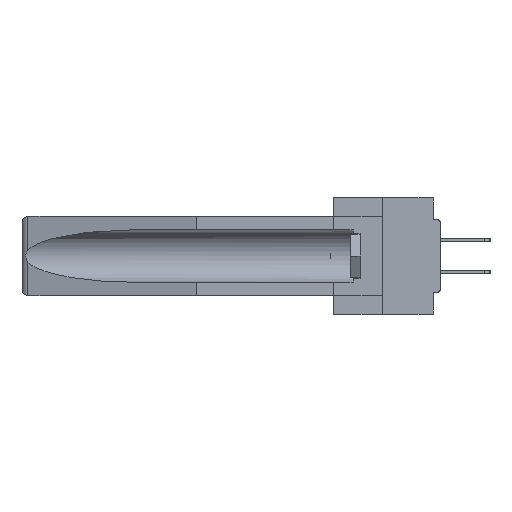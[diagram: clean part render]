
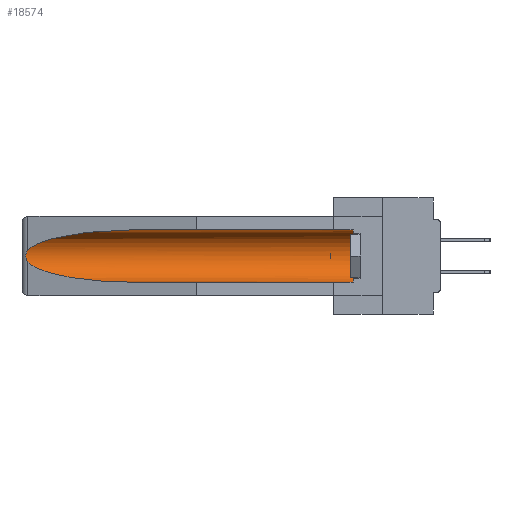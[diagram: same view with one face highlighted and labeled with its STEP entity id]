
A CAD part, left-side view. The second image highlights one B-rep face of the part: STEP entity #18574.
In plain terms, the highlighted cylindrical face has radius 2.857 mm (diameter 5.715 mm), a partial arc.
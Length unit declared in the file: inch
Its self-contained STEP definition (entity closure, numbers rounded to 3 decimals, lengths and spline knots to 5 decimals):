
#518 = CARTESIAN_POINT ( 'NONE',  ( 0.2675, 1.53308, -0.17534 ) ) ;
#885 =( BOUNDED_CURVE ( )  B_SPLINE_CURVE ( 3, ( #21315, #24932, #2409, #2583 ),
 .UNSPECIFIED., .F., .F. ) 
 B_SPLINE_CURVE_WITH_KNOTS ( ( 4, 4 ),
 ( 0.1948, 1.5708 ),
 .UNSPECIFIED. ) 
 CURVE ( )  GEOMETRIC_REPRESENTATION_ITEM ( )  RATIONAL_B_SPLINE_CURVE ( ( 1., 0.848, 0.848, 1. ) ) 
 REPRESENTATION_ITEM ( '' )  );
#930 = CARTESIAN_POINT ( 'NONE',  ( 0.26537, 1.52718, -0.19328 ) ) ;
#1600 = ORIENTED_EDGE ( 'NONE', *, *, #28235, .T. ) ;
#1963 = CYLINDRICAL_SURFACE ( 'NONE', #11895, 0.1125 ) ;
#2409 = CARTESIAN_POINT ( 'NONE',  ( 0.21114, 1.30732, -0.284 ) ) ;
#2583 = CARTESIAN_POINT ( 'NONE',  ( 0.155, 1.07973, -0.284 ) ) ;
#4950 = ORIENTED_EDGE ( 'NONE', *, *, #33860, .T. ) ;
#4964 = VERTEX_POINT ( 'NONE', #39233 ) ;
#5385 = B_SPLINE_CURVE_WITH_KNOTS ( 'NONE', 3,
 ( #12181, #19436, #42300, #22942, #45611, #518, #8095, #34482, #15818, #11859 ),
 .UNSPECIFIED., .F., .F.,
 ( 4, 2, 2, 2, 4 ),
 ( 0., 0.00029, 0.00058, 0.00087, 0.00117 ),
 .UNSPECIFIED. ) ;
#6001 = DIRECTION ( 'NONE',  ( 0., 0., 1. ) ) ;
#6864 = VERTEX_POINT ( 'NONE', #9263 ) ;
#7170 = VERTEX_POINT ( 'NONE', #33007 ) ;
#7695 = CARTESIAN_POINT ( 'NONE',  ( 0.155, 1.07973, -0.059 ) ) ;
#8095 = CARTESIAN_POINT ( 'NONE',  ( 0.2673, 1.53269, -0.17917 ) ) ;
#9210 = VECTOR ( 'NONE', #47392, 39.37008 ) ;
#9263 = CARTESIAN_POINT ( 'NONE',  ( 0.155, 1.07973, -0.059 ) ) ;
#10290 = DIRECTION ( 'NONE',  ( 0., 0., 1. ) ) ;
#11093 = VERTEX_POINT ( 'NONE', #930 ) ;
#11859 = CARTESIAN_POINT ( 'NONE',  ( 0.26537, 1.52718, -0.19328 ) ) ;
#11895 = AXIS2_PLACEMENT_3D ( 'NONE', #39595, #17038, #6001 ) ;
#12181 = CARTESIAN_POINT ( 'NONE',  ( 0.26537, 1.52718, -0.14972 ) ) ;
#13840 = EDGE_CURVE ( 'NONE', #7170, #28774, #37529, .T. ) ;
#14205 = EDGE_CURVE ( 'NONE', #4964, #11093, #5385, .T. ) ;
#14772 =( BOUNDED_CURVE ( )  B_SPLINE_CURVE ( 3, ( #7695, #41746, #44884, #23325 ),
 .UNSPECIFIED., .F., .F. ) 
 B_SPLINE_CURVE_WITH_KNOTS ( ( 4, 4 ),
 ( 4.71239, 6.08839 ),
 .UNSPECIFIED. ) 
 CURVE ( )  GEOMETRIC_REPRESENTATION_ITEM ( )  RATIONAL_B_SPLINE_CURVE ( ( 1., 0.848, 0.848, 1. ) ) 
 REPRESENTATION_ITEM ( '' )  );
#15818 = CARTESIAN_POINT ( 'NONE',  ( 0.26597, 1.5296, -0.19026 ) ) ;
#17038 = DIRECTION ( 'NONE',  ( 0., 1., 0. ) ) ;
#17733 = DIRECTION ( 'NONE',  ( 0., -1., 0. ) ) ;
#18574 = ADVANCED_FACE ( 'NONE', ( #21988 ), #1963, .F. ) ;
#18771 = DIRECTION ( 'NONE',  ( 0., 1., 0. ) ) ;
#19436 = CARTESIAN_POINT ( 'NONE',  ( 0.26597, 1.52961, -0.15275 ) ) ;
#19965 = ORIENTED_EDGE ( 'NONE', *, *, #14205, .T. ) ;
#21315 = CARTESIAN_POINT ( 'NONE',  ( 0.26537, 1.52718, -0.19328 ) ) ;
#21988 = FACE_OUTER_BOUND ( 'NONE', #35170, .T. ) ;
#22942 = CARTESIAN_POINT ( 'NONE',  ( 0.2673, 1.5327, -0.16383 ) ) ;
#23325 = CARTESIAN_POINT ( 'NONE',  ( 0.26537, 1.52718, -0.14972 ) ) ;
#24809 = EDGE_CURVE ( 'NONE', #6864, #4964, #14772, .T. ) ;
#24932 = CARTESIAN_POINT ( 'NONE',  ( 0.25451, 1.48313, -0.24835 ) ) ;
#25028 = VERTEX_POINT ( 'NONE', #47163 ) ;
#25166 = EDGE_CURVE ( 'NONE', #7170, #25028, #32384, .T. ) ;
#25297 = CARTESIAN_POINT ( 'NONE',  ( 0.155, 0.126, -0.1715 ) ) ;
#25454 = AXIS2_PLACEMENT_3D ( 'NONE', #25297, #17733, #10290 ) ;
#28235 = EDGE_CURVE ( 'NONE', #25028, #6864, #39271, .T. ) ;
#28774 = VERTEX_POINT ( 'NONE', #36506 ) ;
#29211 = ORIENTED_EDGE ( 'NONE', *, *, #25166, .T. ) ;
#32384 = CIRCLE ( 'NONE', #25454, 0.1125 ) ;
#33007 = CARTESIAN_POINT ( 'NONE',  ( 0.155, 0.126, -0.284 ) ) ;
#33860 = EDGE_CURVE ( 'NONE', #11093, #28774, #885, .T. ) ;
#33957 = CARTESIAN_POINT ( 'NONE',  ( 0.155, -0.30754, -0.284 ) ) ;
#34482 = CARTESIAN_POINT ( 'NONE',  ( 0.26655, 1.53094, -0.18657 ) ) ;
#35170 = EDGE_LOOP ( 'NONE', ( #48294, #19965, #4950, #39184, #29211, #1600 ) ) ;
#36506 = CARTESIAN_POINT ( 'NONE',  ( 0.155, 1.07973, -0.284 ) ) ;
#37529 = LINE ( 'NONE', #33957, #43991 ) ;
#39184 = ORIENTED_EDGE ( 'NONE', *, *, #13840, .F. ) ;
#39233 = CARTESIAN_POINT ( 'NONE',  ( 0.26537, 1.52718, -0.14972 ) ) ;
#39271 = LINE ( 'NONE', #43772, #9210 ) ;
#39595 = CARTESIAN_POINT ( 'NONE',  ( 0.155, -0.30754, -0.1715 ) ) ;
#41746 = CARTESIAN_POINT ( 'NONE',  ( 0.21114, 1.30732, -0.059 ) ) ;
#42300 = CARTESIAN_POINT ( 'NONE',  ( 0.26654, 1.53092, -0.15636 ) ) ;
#43772 = CARTESIAN_POINT ( 'NONE',  ( 0.155, -0.30754, -0.059 ) ) ;
#43991 = VECTOR ( 'NONE', #18771, 39.37008 ) ;
#44884 = CARTESIAN_POINT ( 'NONE',  ( 0.25451, 1.48313, -0.09465 ) ) ;
#45611 = CARTESIAN_POINT ( 'NONE',  ( 0.2675, 1.53308, -0.16763 ) ) ;
#47163 = CARTESIAN_POINT ( 'NONE',  ( 0.155, 0.126, -0.059 ) ) ;
#47392 = DIRECTION ( 'NONE',  ( 0., 1., 0. ) ) ;
#48294 = ORIENTED_EDGE ( 'NONE', *, *, #24809, .T. ) ;
